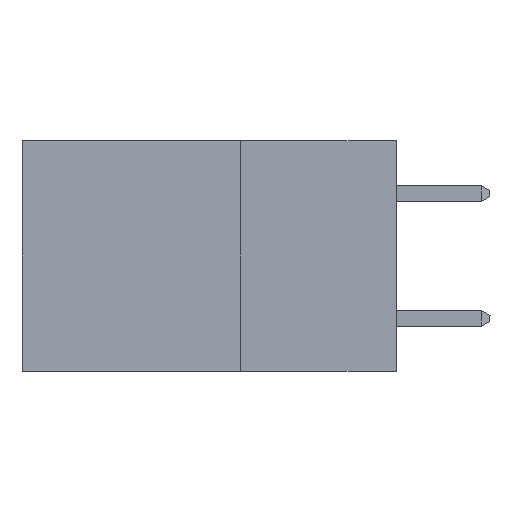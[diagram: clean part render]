
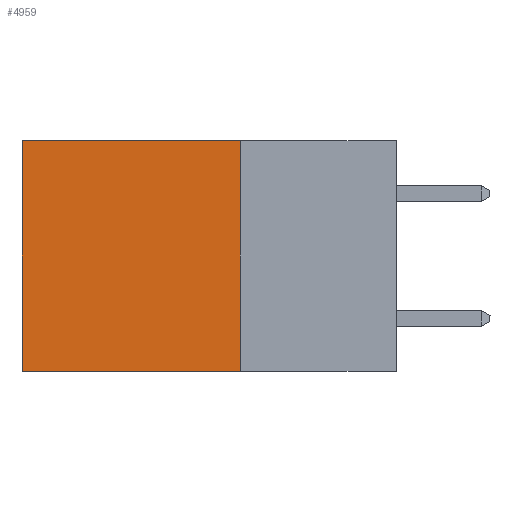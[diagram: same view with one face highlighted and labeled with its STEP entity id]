
A CAD part, left-side view. The second image highlights one B-rep face of the part: STEP entity #4959.
In plain terms, the highlighted planar face has unit normal (-1, 0, 0).
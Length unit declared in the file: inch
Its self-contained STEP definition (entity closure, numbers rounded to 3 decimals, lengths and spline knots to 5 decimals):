
#3464 = CARTESIAN_POINT ( 'NONE',  ( 0.298, 0.25, 0. ) ) ;
#3689 = EDGE_LOOP ( 'NONE', ( #9082, #11840, #21182, #16907 ) ) ;
#4441 = VECTOR ( 'NONE', #9188, 39.37008 ) ;
#4507 = CARTESIAN_POINT ( 'NONE',  ( 0.298, 0.25, -0.37 ) ) ;
#4603 = EDGE_CURVE ( 'NONE', #10849, #5598, #22925, .T. ) ;
#4959 = ADVANCED_FACE ( 'NONE', ( #19355 ), #16461, .F. ) ;
#5598 = VERTEX_POINT ( 'NONE', #20309 ) ;
#5788 = VERTEX_POINT ( 'NONE', #4507 ) ;
#6552 = VERTEX_POINT ( 'NONE', #8375 ) ;
#7428 = DIRECTION ( 'NONE',  ( 0., 1., 0. ) ) ;
#8375 = CARTESIAN_POINT ( 'NONE',  ( 0.298, 0.6, -0.37 ) ) ;
#9082 = ORIENTED_EDGE ( 'NONE', *, *, #10096, .T. ) ;
#9188 = DIRECTION ( 'NONE',  ( 0., 1., 0. ) ) ;
#10096 = EDGE_CURVE ( 'NONE', #5598, #6552, #24150, .T. ) ;
#10242 = DIRECTION ( 'NONE',  ( 1., 0., 0. ) ) ;
#10849 = VERTEX_POINT ( 'NONE', #15550 ) ;
#11840 = ORIENTED_EDGE ( 'NONE', *, *, #16816, .F. ) ;
#11975 = VECTOR ( 'NONE', #24766, 39.37008 ) ;
#13830 = VECTOR ( 'NONE', #7428, 39.37008 ) ;
#15166 = DIRECTION ( 'NONE',  ( 0., 0., -1. ) ) ;
#15550 = CARTESIAN_POINT ( 'NONE',  ( 0.298, 0.25, 0. ) ) ;
#15916 = AXIS2_PLACEMENT_3D ( 'NONE', #22825, #10242, #24715 ) ;
#16461 = PLANE ( 'NONE',  #15916 ) ;
#16816 = EDGE_CURVE ( 'NONE', #5788, #6552, #25438, .T. ) ;
#16907 = ORIENTED_EDGE ( 'NONE', *, *, #4603, .T. ) ;
#19309 = CARTESIAN_POINT ( 'NONE',  ( 0.298, 0.25, -0.37 ) ) ;
#19355 = FACE_OUTER_BOUND ( 'NONE', #3689, .T. ) ;
#19464 = EDGE_CURVE ( 'NONE', #10849, #5788, #25595, .T. ) ;
#19657 = CARTESIAN_POINT ( 'NONE',  ( 0.298, 0.6, 0. ) ) ;
#20309 = CARTESIAN_POINT ( 'NONE',  ( 0.298, 0.6, 0. ) ) ;
#21182 = ORIENTED_EDGE ( 'NONE', *, *, #19464, .F. ) ;
#22695 = CARTESIAN_POINT ( 'NONE',  ( 0.298, 0.25, 0. ) ) ;
#22825 = CARTESIAN_POINT ( 'NONE',  ( 0.298, 0.25, 0. ) ) ;
#22925 = LINE ( 'NONE', #3464, #13830 ) ;
#24150 = LINE ( 'NONE', #19657, #25729 ) ;
#24715 = DIRECTION ( 'NONE',  ( 0., 0., -1. ) ) ;
#24766 = DIRECTION ( 'NONE',  ( 0., 0., -1. ) ) ;
#25438 = LINE ( 'NONE', #19309, #4441 ) ;
#25595 = LINE ( 'NONE', #22695, #11975 ) ;
#25729 = VECTOR ( 'NONE', #15166, 39.37008 ) ;
